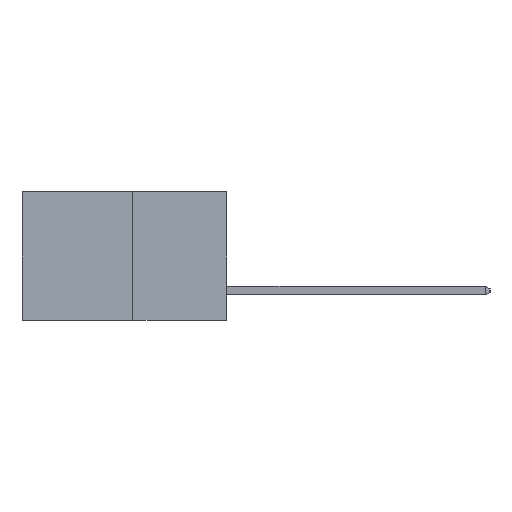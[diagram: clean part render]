
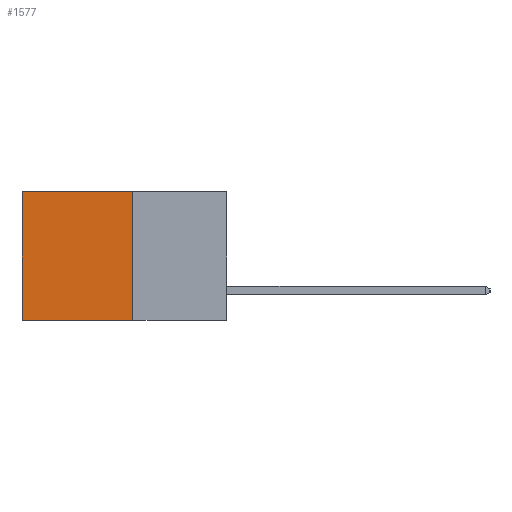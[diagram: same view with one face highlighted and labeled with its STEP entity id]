
A CAD part, left-side view. The second image highlights one B-rep face of the part: STEP entity #1577.
In plain terms, the highlighted planar face has unit normal (-1, 0, 0).
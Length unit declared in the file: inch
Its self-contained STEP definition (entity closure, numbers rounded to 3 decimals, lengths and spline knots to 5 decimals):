
#343 = VECTOR ( 'NONE', #6332, 39.37008 ) ;
#571 = CARTESIAN_POINT ( 'NONE',  ( 0.277, 0.27, 0. ) ) ;
#740 = ORIENTED_EDGE ( 'NONE', *, *, #8748, .F. ) ;
#1577 = ADVANCED_FACE ( 'NONE', ( #5022 ), #2000, .F. ) ;
#2000 = PLANE ( 'NONE',  #2625 ) ;
#2625 = AXIS2_PLACEMENT_3D ( 'NONE', #9683, #7790, #8456 ) ;
#2642 = LINE ( 'NONE', #571, #6601 ) ;
#3047 = CARTESIAN_POINT ( 'NONE',  ( 0.277, 0.59, 0. ) ) ;
#3894 = DIRECTION ( 'NONE',  ( 0., 0., -1. ) ) ;
#4194 = CARTESIAN_POINT ( 'NONE',  ( 0.277, 0.27, -0.37 ) ) ;
#4971 = VERTEX_POINT ( 'NONE', #6140 ) ;
#4997 = VERTEX_POINT ( 'NONE', #6094 ) ;
#5022 = FACE_OUTER_BOUND ( 'NONE', #10606, .T. ) ;
#5437 = ORIENTED_EDGE ( 'NONE', *, *, #10812, .F. ) ;
#5529 = CARTESIAN_POINT ( 'NONE',  ( 0.277, 0.27, -0.37 ) ) ;
#6094 = CARTESIAN_POINT ( 'NONE',  ( 0.277, 0.59, -0.37 ) ) ;
#6140 = CARTESIAN_POINT ( 'NONE',  ( 0.277, 0.27, 0. ) ) ;
#6332 = DIRECTION ( 'NONE',  ( 0., 1., 0. ) ) ;
#6601 = VECTOR ( 'NONE', #6651, 39.37008 ) ;
#6651 = DIRECTION ( 'NONE',  ( 0., 1., 0. ) ) ;
#6702 = CARTESIAN_POINT ( 'NONE',  ( 0.277, 0.27, -0.37 ) ) ;
#7128 = VERTEX_POINT ( 'NONE', #3047 ) ;
#7259 = LINE ( 'NONE', #5529, #343 ) ;
#7614 = ORIENTED_EDGE ( 'NONE', *, *, #9120, .T. ) ;
#7790 = DIRECTION ( 'NONE',  ( 1., 0., 0. ) ) ;
#7987 = CARTESIAN_POINT ( 'NONE',  ( 0.277, 0.59, -0.37 ) ) ;
#8383 = VECTOR ( 'NONE', #10671, 39.37008 ) ;
#8456 = DIRECTION ( 'NONE',  ( 0., 0., -1. ) ) ;
#8638 = LINE ( 'NONE', #6702, #8383 ) ;
#8748 = EDGE_CURVE ( 'NONE', #9945, #4997, #7259, .T. ) ;
#9120 = EDGE_CURVE ( 'NONE', #4971, #7128, #2642, .T. ) ;
#9533 = VECTOR ( 'NONE', #3894, 39.37008 ) ;
#9537 = ORIENTED_EDGE ( 'NONE', *, *, #10459, .T. ) ;
#9683 = CARTESIAN_POINT ( 'NONE',  ( 0.277, 0.27, -0.37 ) ) ;
#9781 = LINE ( 'NONE', #7987, #9533 ) ;
#9945 = VERTEX_POINT ( 'NONE', #4194 ) ;
#10459 = EDGE_CURVE ( 'NONE', #7128, #4997, #9781, .T. ) ;
#10606 = EDGE_LOOP ( 'NONE', ( #9537, #740, #5437, #7614 ) ) ;
#10671 = DIRECTION ( 'NONE',  ( 0., 0., -1. ) ) ;
#10812 = EDGE_CURVE ( 'NONE', #4971, #9945, #8638, .T. ) ;
